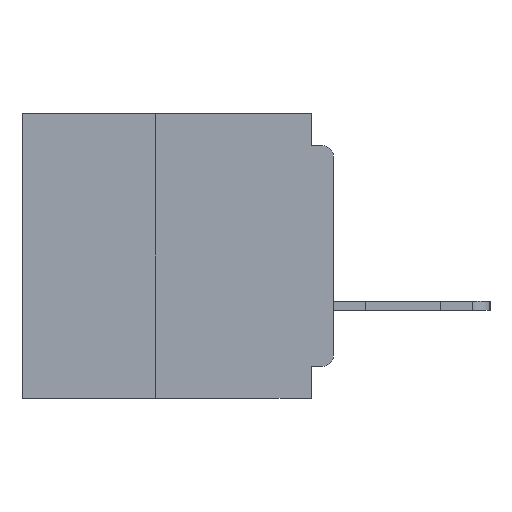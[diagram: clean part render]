
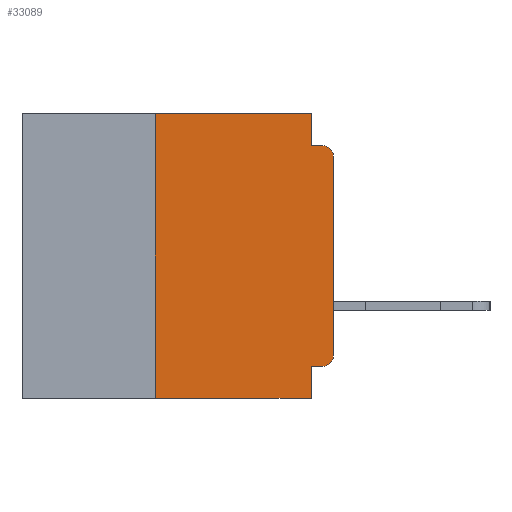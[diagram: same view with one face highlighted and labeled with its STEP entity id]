
A CAD part, left-side view. The second image highlights one B-rep face of the part: STEP entity #33089.
In plain terms, the highlighted planar face has unit normal (-1, 0, 0).
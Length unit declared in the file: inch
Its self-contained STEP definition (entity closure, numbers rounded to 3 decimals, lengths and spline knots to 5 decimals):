
#14 = ORIENTED_EDGE ( 'NONE', *, *, #6894, .F. ) ;
#461 = DIRECTION ( 'NONE',  ( 0., 0., -1. ) ) ;
#745 = CARTESIAN_POINT ( 'NONE',  ( 0., 0.25, 0. ) ) ;
#1572 = VERTEX_POINT ( 'NONE', #18487 ) ;
#1682 = CARTESIAN_POINT ( 'NONE',  ( 0., 0., -0.34 ) ) ;
#1888 = EDGE_CURVE ( 'NONE', #1572, #7239, #26928, .T. ) ;
#2092 = VECTOR ( 'NONE', #46724, 39.37008 ) ;
#2220 = VECTOR ( 'NONE', #14102, 39.37008 ) ;
#2256 = AXIS2_PLACEMENT_3D ( 'NONE', #35382, #13054, #39130 ) ;
#2374 = ORIENTED_EDGE ( 'NONE', *, *, #4766, .F. ) ;
#2508 = ORIENTED_EDGE ( 'NONE', *, *, #29812, .F. ) ;
#4068 = VERTEX_POINT ( 'NONE', #29943 ) ;
#4394 = EDGE_CURVE ( 'NONE', #5824, #7239, #46557, .T. ) ;
#4766 = EDGE_CURVE ( 'NONE', #12007, #1572, #21457, .T. ) ;
#5824 = VERTEX_POINT ( 'NONE', #48355 ) ;
#6894 = EDGE_CURVE ( 'NONE', #5824, #43233, #39887, .T. ) ;
#7239 = VERTEX_POINT ( 'NONE', #11039 ) ;
#7557 = CARTESIAN_POINT ( 'NONE',  ( 0., 0.015, -0.06 ) ) ;
#7829 = CARTESIAN_POINT ( 'NONE',  ( 0., 0., -0.355 ) ) ;
#10282 = CARTESIAN_POINT ( 'NONE',  ( 0., 0., -0.045 ) ) ;
#10328 = VECTOR ( 'NONE', #19149, 39.37008 ) ;
#11039 = CARTESIAN_POINT ( 'NONE',  ( 0., 0.031, -0.4 ) ) ;
#11222 = VERTEX_POINT ( 'NONE', #42223 ) ;
#11352 = DIRECTION ( 'NONE',  ( 0., 0., -1. ) ) ;
#11378 = EDGE_CURVE ( 'NONE', #23160, #11222, #33079, .T. ) ;
#11964 = ORIENTED_EDGE ( 'NONE', *, *, #11378, .T. ) ;
#12007 = VERTEX_POINT ( 'NONE', #47486 ) ;
#13054 = DIRECTION ( 'NONE',  ( 1., 0., 0. ) ) ;
#13179 = ORIENTED_EDGE ( 'NONE', *, *, #48196, .T. ) ;
#13556 = LINE ( 'NONE', #17300, #32191 ) ;
#14102 = DIRECTION ( 'NONE',  ( 0., -1., 0. ) ) ;
#14701 = AXIS2_PLACEMENT_3D ( 'NONE', #7557, #33702, #11352 ) ;
#14841 = CIRCLE ( 'NONE', #14701, 0.015 ) ;
#15920 = ORIENTED_EDGE ( 'NONE', *, *, #35769, .T. ) ;
#16524 = CARTESIAN_POINT ( 'NONE',  ( 0., 0.25, -0.4 ) ) ;
#17011 = EDGE_CURVE ( 'NONE', #20519, #32351, #13556, .T. ) ;
#17300 = CARTESIAN_POINT ( 'NONE',  ( 0., 0.031, 0. ) ) ;
#18487 = CARTESIAN_POINT ( 'NONE',  ( 0., 0.031, -0.355 ) ) ;
#19149 = DIRECTION ( 'NONE',  ( 0., 1., 0. ) ) ;
#19711 = ORIENTED_EDGE ( 'NONE', *, *, #37411, .F. ) ;
#20086 = VECTOR ( 'NONE', #20247, 39.37008 ) ;
#20247 = DIRECTION ( 'NONE',  ( 0., 0., 1. ) ) ;
#20519 = VERTEX_POINT ( 'NONE', #38780 ) ;
#20663 = DIRECTION ( 'NONE',  ( 0., -1., 0. ) ) ;
#21044 = DIRECTION ( 'NONE',  ( 0., 0., -1. ) ) ;
#21294 = DIRECTION ( 'NONE',  ( 0., -1., 0. ) ) ;
#21359 = ORIENTED_EDGE ( 'NONE', *, *, #4394, .T. ) ;
#21457 = LINE ( 'NONE', #7829, #10328 ) ;
#22877 = DIRECTION ( 'NONE',  ( -1., 0., 0. ) ) ;
#23160 = VERTEX_POINT ( 'NONE', #1682 ) ;
#24113 = PLANE ( 'NONE',  #2256 ) ;
#24372 = VECTOR ( 'NONE', #21294, 39.37008 ) ;
#25745 = VECTOR ( 'NONE', #40386, 39.37008 ) ;
#26903 = CIRCLE ( 'NONE', #39884, 0.015 ) ;
#26928 = LINE ( 'NONE', #42706, #25745 ) ;
#29812 = EDGE_CURVE ( 'NONE', #32351, #4068, #32063, .T. ) ;
#29943 = CARTESIAN_POINT ( 'NONE',  ( 0., 0.015, -0.045 ) ) ;
#30866 = ORIENTED_EDGE ( 'NONE', *, *, #17011, .F. ) ;
#31875 = CARTESIAN_POINT ( 'NONE',  ( 0., 0.437, -0.4 ) ) ;
#31921 = CARTESIAN_POINT ( 'NONE',  ( 0., 0., 0. ) ) ;
#32063 = LINE ( 'NONE', #10282, #2220 ) ;
#32191 = VECTOR ( 'NONE', #21044, 39.37008 ) ;
#32351 = VERTEX_POINT ( 'NONE', #38228 ) ;
#32362 = CARTESIAN_POINT ( 'NONE',  ( 0., 0.437, 0. ) ) ;
#33079 = LINE ( 'NONE', #31921, #2092 ) ;
#33089 = ADVANCED_FACE ( 'NONE', ( #46262 ), #24113, .F. ) ;
#33702 = DIRECTION ( 'NONE',  ( -1., 0., 0. ) ) ;
#35097 = ORIENTED_EDGE ( 'NONE', *, *, #1888, .F. ) ;
#35382 = CARTESIAN_POINT ( 'NONE',  ( 0., 0.437, 0. ) ) ;
#35489 = LINE ( 'NONE', #32362, #24372 ) ;
#35769 = EDGE_CURVE ( 'NONE', #12007, #23160, #26903, .T. ) ;
#36665 = VECTOR ( 'NONE', #20663, 39.37008 ) ;
#37411 = EDGE_CURVE ( 'NONE', #43233, #20519, #35489, .T. ) ;
#38228 = CARTESIAN_POINT ( 'NONE',  ( 0., 0.031, -0.045 ) ) ;
#38780 = CARTESIAN_POINT ( 'NONE',  ( 0., 0.031, 0. ) ) ;
#39130 = DIRECTION ( 'NONE',  ( 0., 0., -1. ) ) ;
#39884 = AXIS2_PLACEMENT_3D ( 'NONE', #45192, #22877, #461 ) ;
#39887 = LINE ( 'NONE', #16524, #20086 ) ;
#40386 = DIRECTION ( 'NONE',  ( 0., 0., -1. ) ) ;
#42223 = CARTESIAN_POINT ( 'NONE',  ( 0., 0., -0.06 ) ) ;
#42706 = CARTESIAN_POINT ( 'NONE',  ( 0., 0.031, -0.4 ) ) ;
#43233 = VERTEX_POINT ( 'NONE', #745 ) ;
#44693 = EDGE_LOOP ( 'NONE', ( #11964, #13179, #2508, #30866, #19711, #14, #21359, #35097, #2374, #15920 ) ) ;
#45192 = CARTESIAN_POINT ( 'NONE',  ( 0., 0.015, -0.34 ) ) ;
#46262 = FACE_OUTER_BOUND ( 'NONE', #44693, .T. ) ;
#46557 = LINE ( 'NONE', #31875, #36665 ) ;
#46724 = DIRECTION ( 'NONE',  ( 0., 0., 1. ) ) ;
#47486 = CARTESIAN_POINT ( 'NONE',  ( 0., 0.015, -0.355 ) ) ;
#48196 = EDGE_CURVE ( 'NONE', #11222, #4068, #14841, .T. ) ;
#48355 = CARTESIAN_POINT ( 'NONE',  ( 0., 0.25, -0.4 ) ) ;
